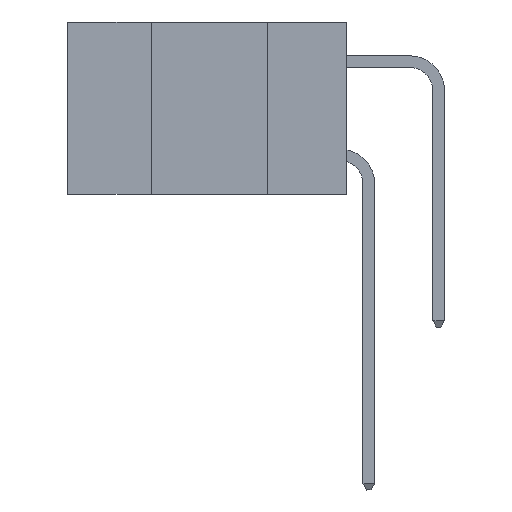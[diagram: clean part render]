
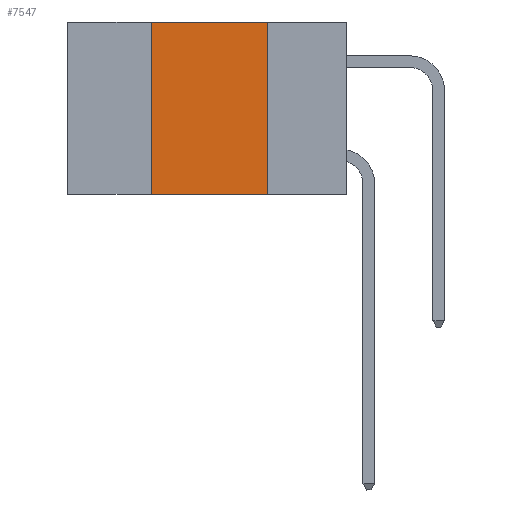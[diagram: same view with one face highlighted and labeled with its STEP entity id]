
A CAD part, left-side view. The second image highlights one B-rep face of the part: STEP entity #7547.
In plain terms, the highlighted planar face has unit normal (-1, 0, 0).
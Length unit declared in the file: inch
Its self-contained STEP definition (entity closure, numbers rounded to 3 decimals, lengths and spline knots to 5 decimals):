
#170 = CARTESIAN_POINT ( 'NONE',  ( 0., 0.42, 0. ) ) ;
#982 = VECTOR ( 'NONE', #7573, 39.37008 ) ;
#1085 = LINE ( 'NONE', #14899, #13018 ) ;
#2264 = EDGE_CURVE ( 'NONE', #15256, #3074, #7060, .T. ) ;
#2392 = PLANE ( 'NONE',  #4008 ) ;
#2464 = LINE ( 'NONE', #10891, #11863 ) ;
#3074 = VERTEX_POINT ( 'NONE', #10528 ) ;
#3373 = EDGE_LOOP ( 'NONE', ( #7750, #8820, #4848, #5120 ) ) ;
#4008 = AXIS2_PLACEMENT_3D ( 'NONE', #12562, #14949, #8650 ) ;
#4171 = FACE_OUTER_BOUND ( 'NONE', #3373, .T. ) ;
#4631 = LINE ( 'NONE', #14090, #982 ) ;
#4661 = CARTESIAN_POINT ( 'NONE',  ( 0., 0.42, -0.37 ) ) ;
#4848 = ORIENTED_EDGE ( 'NONE', *, *, #5271, .F. ) ;
#5120 = ORIENTED_EDGE ( 'NONE', *, *, #9196, .T. ) ;
#5271 = EDGE_CURVE ( 'NONE', #11800, #15256, #4631, .T. ) ;
#5548 = VERTEX_POINT ( 'NONE', #14477 ) ;
#7060 = LINE ( 'NONE', #14313, #15686 ) ;
#7547 = ADVANCED_FACE ( 'NONE', ( #4171 ), #2392, .F. ) ;
#7573 = DIRECTION ( 'NONE',  ( 0., 0., 1. ) ) ;
#7750 = ORIENTED_EDGE ( 'NONE', *, *, #13632, .F. ) ;
#8650 = DIRECTION ( 'NONE',  ( 0., 0., -1. ) ) ;
#8755 = DIRECTION ( 'NONE',  ( 0., 0., -1. ) ) ;
#8820 = ORIENTED_EDGE ( 'NONE', *, *, #2264, .F. ) ;
#9196 = EDGE_CURVE ( 'NONE', #11800, #5548, #2464, .T. ) ;
#10528 = CARTESIAN_POINT ( 'NONE',  ( 0., 0.17, 0. ) ) ;
#10891 = CARTESIAN_POINT ( 'NONE',  ( 0., 0.6, -0.37 ) ) ;
#11800 = VERTEX_POINT ( 'NONE', #4661 ) ;
#11863 = VECTOR ( 'NONE', #15792, 39.37008 ) ;
#11989 = DIRECTION ( 'NONE',  ( 0., -1., 0. ) ) ;
#12562 = CARTESIAN_POINT ( 'NONE',  ( 0., 0.6, 0. ) ) ;
#13018 = VECTOR ( 'NONE', #8755, 39.37008 ) ;
#13632 = EDGE_CURVE ( 'NONE', #3074, #5548, #1085, .T. ) ;
#14090 = CARTESIAN_POINT ( 'NONE',  ( 0., 0.42, 0. ) ) ;
#14313 = CARTESIAN_POINT ( 'NONE',  ( 0., 0.6, 0. ) ) ;
#14477 = CARTESIAN_POINT ( 'NONE',  ( 0., 0.17, -0.37 ) ) ;
#14899 = CARTESIAN_POINT ( 'NONE',  ( 0., 0.17, 0. ) ) ;
#14949 = DIRECTION ( 'NONE',  ( 1., 0., 0. ) ) ;
#15256 = VERTEX_POINT ( 'NONE', #170 ) ;
#15686 = VECTOR ( 'NONE', #11989, 39.37008 ) ;
#15792 = DIRECTION ( 'NONE',  ( 0., -1., 0. ) ) ;
